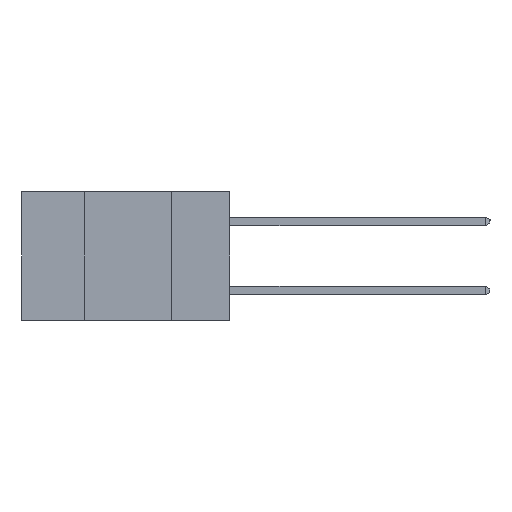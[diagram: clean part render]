
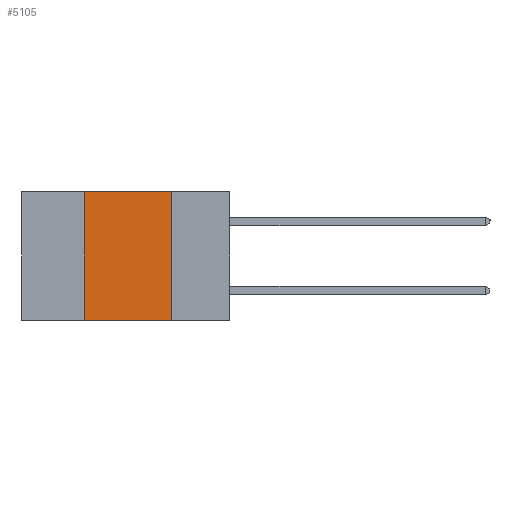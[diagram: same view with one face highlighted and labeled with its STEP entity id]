
A CAD part, left-side view. The second image highlights one B-rep face of the part: STEP entity #5105.
In plain terms, the highlighted planar face has unit normal (-1, 0, 0).
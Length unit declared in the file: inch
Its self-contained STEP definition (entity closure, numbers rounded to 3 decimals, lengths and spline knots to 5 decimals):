
#966 = CARTESIAN_POINT ( 'NONE',  ( 0., 0.6, 0. ) ) ;
#1262 = EDGE_CURVE ( 'NONE', #3544, #6395, #2179, .T. ) ;
#1684 = EDGE_CURVE ( 'NONE', #6395, #5267, #8557, .T. ) ;
#2152 = EDGE_CURVE ( 'NONE', #11680, #5267, #9712, .T. ) ;
#2179 = LINE ( 'NONE', #966, #6840 ) ;
#2943 = ORIENTED_EDGE ( 'NONE', *, *, #1684, .F. ) ;
#3544 = VERTEX_POINT ( 'NONE', #5326 ) ;
#4105 = CARTESIAN_POINT ( 'NONE',  ( 0., 0.42, -0.37 ) ) ;
#4729 = CARTESIAN_POINT ( 'NONE',  ( 0., 0.17, -0.37 ) ) ;
#4817 = DIRECTION ( 'NONE',  ( 0., -1., 0. ) ) ;
#5105 = ADVANCED_FACE ( 'NONE', ( #12950 ), #9148, .F. ) ;
#5256 = CARTESIAN_POINT ( 'NONE',  ( 0., 0.42, -0.37 ) ) ;
#5267 = VERTEX_POINT ( 'NONE', #10968 ) ;
#5326 = CARTESIAN_POINT ( 'NONE',  ( 0., 0.42, 0. ) ) ;
#5608 = ORIENTED_EDGE ( 'NONE', *, *, #2152, .T. ) ;
#5780 = DIRECTION ( 'NONE',  ( 0., -1., 0. ) ) ;
#5983 = EDGE_LOOP ( 'NONE', ( #2943, #16007, #8269, #5608 ) ) ;
#6395 = VERTEX_POINT ( 'NONE', #13885 ) ;
#6709 = VECTOR ( 'NONE', #8137, 39.37008 ) ;
#6840 = VECTOR ( 'NONE', #4817, 39.37008 ) ;
#8137 = DIRECTION ( 'NONE',  ( 0., 0., 1. ) ) ;
#8269 = ORIENTED_EDGE ( 'NONE', *, *, #15974, .F. ) ;
#8557 = LINE ( 'NONE', #4729, #12848 ) ;
#9006 = VECTOR ( 'NONE', #5780, 39.37008 ) ;
#9148 = PLANE ( 'NONE',  #11810 ) ;
#9712 = LINE ( 'NONE', #12277, #9006 ) ;
#10968 = CARTESIAN_POINT ( 'NONE',  ( 0., 0.17, -0.37 ) ) ;
#10981 = DIRECTION ( 'NONE',  ( 0., 0., -1. ) ) ;
#11654 = DIRECTION ( 'NONE',  ( 1., 0., 0. ) ) ;
#11680 = VERTEX_POINT ( 'NONE', #4105 ) ;
#11760 = LINE ( 'NONE', #5256, #6709 ) ;
#11810 = AXIS2_PLACEMENT_3D ( 'NONE', #16770, #11654, #14297 ) ;
#12277 = CARTESIAN_POINT ( 'NONE',  ( 0., 0.6, -0.37 ) ) ;
#12848 = VECTOR ( 'NONE', #10981, 39.37008 ) ;
#12950 = FACE_OUTER_BOUND ( 'NONE', #5983, .T. ) ;
#13885 = CARTESIAN_POINT ( 'NONE',  ( 0., 0.17, 0. ) ) ;
#14297 = DIRECTION ( 'NONE',  ( 0., 0., -1. ) ) ;
#15974 = EDGE_CURVE ( 'NONE', #11680, #3544, #11760, .T. ) ;
#16007 = ORIENTED_EDGE ( 'NONE', *, *, #1262, .F. ) ;
#16770 = CARTESIAN_POINT ( 'NONE',  ( 0., 0.6, 0. ) ) ;
